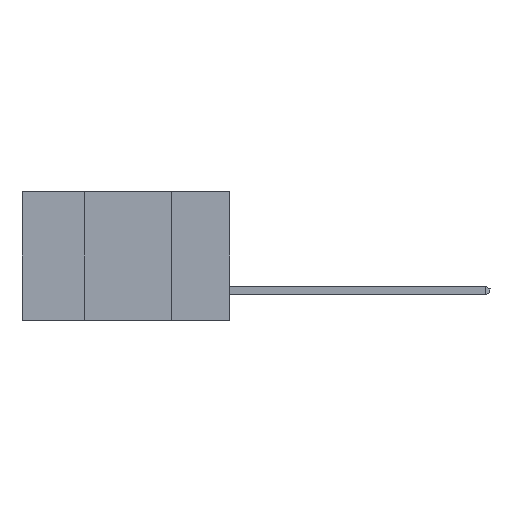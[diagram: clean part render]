
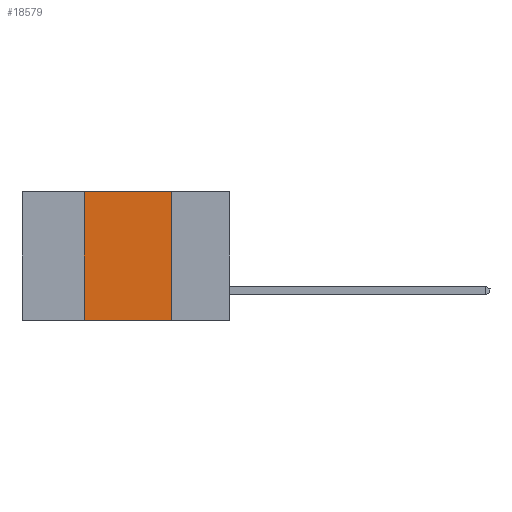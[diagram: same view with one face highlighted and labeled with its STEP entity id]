
A CAD part, left-side view. The second image highlights one B-rep face of the part: STEP entity #18579.
In plain terms, the highlighted planar face has unit normal (-1, 0, 0).
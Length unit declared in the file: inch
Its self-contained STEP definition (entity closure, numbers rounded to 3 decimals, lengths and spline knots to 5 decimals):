
#257 = FACE_OUTER_BOUND ( 'NONE', #25144, .T. ) ;
#737 = CARTESIAN_POINT ( 'NONE',  ( 0., 0.6, -0.37 ) ) ;
#833 = LINE ( 'NONE', #20467, #21780 ) ;
#2364 = DIRECTION ( 'NONE',  ( 0., 0., -1. ) ) ;
#2722 = LINE ( 'NONE', #20997, #23050 ) ;
#3212 = CARTESIAN_POINT ( 'NONE',  ( 0., 0.6, 0. ) ) ;
#3334 = DIRECTION ( 'NONE',  ( 0., -1., 0. ) ) ;
#3952 = VERTEX_POINT ( 'NONE', #21026 ) ;
#5825 = CARTESIAN_POINT ( 'NONE',  ( 0., 0.17, 0. ) ) ;
#6505 = CARTESIAN_POINT ( 'NONE',  ( 0., 0.42, -0.37 ) ) ;
#6586 = DIRECTION ( 'NONE',  ( 0., -1., 0. ) ) ;
#8256 = CARTESIAN_POINT ( 'NONE',  ( 0., 0.6, 0. ) ) ;
#10914 = VERTEX_POINT ( 'NONE', #5825 ) ;
#11206 = VERTEX_POINT ( 'NONE', #25024 ) ;
#11713 = AXIS2_PLACEMENT_3D ( 'NONE', #8256, #20779, #2364 ) ;
#12486 = VERTEX_POINT ( 'NONE', #6505 ) ;
#12836 = DIRECTION ( 'NONE',  ( 0., 0., -1. ) ) ;
#14929 = ORIENTED_EDGE ( 'NONE', *, *, #26139, .F. ) ;
#15029 = ORIENTED_EDGE ( 'NONE', *, *, #22091, .T. ) ;
#15104 = DIRECTION ( 'NONE',  ( 0., 0., 1. ) ) ;
#17114 = VECTOR ( 'NONE', #3334, 39.37008 ) ;
#18579 = ADVANCED_FACE ( 'NONE', ( #257 ), #22770, .F. ) ;
#18668 = LINE ( 'NONE', #3212, #17114 ) ;
#19961 = ORIENTED_EDGE ( 'NONE', *, *, #24309, .F. ) ;
#19999 = ORIENTED_EDGE ( 'NONE', *, *, #23776, .F. ) ;
#20467 = CARTESIAN_POINT ( 'NONE',  ( 0., 0.42, -0.37 ) ) ;
#20779 = DIRECTION ( 'NONE',  ( 1., 0., 0. ) ) ;
#20997 = CARTESIAN_POINT ( 'NONE',  ( 0., 0.17, -0.37 ) ) ;
#21001 = LINE ( 'NONE', #737, #22053 ) ;
#21026 = CARTESIAN_POINT ( 'NONE',  ( 0., 0.17, -0.37 ) ) ;
#21780 = VECTOR ( 'NONE', #15104, 39.37008 ) ;
#22053 = VECTOR ( 'NONE', #6586, 39.37008 ) ;
#22091 = EDGE_CURVE ( 'NONE', #12486, #3952, #21001, .T. ) ;
#22770 = PLANE ( 'NONE',  #11713 ) ;
#23050 = VECTOR ( 'NONE', #12836, 39.37008 ) ;
#23776 = EDGE_CURVE ( 'NONE', #12486, #11206, #833, .T. ) ;
#24309 = EDGE_CURVE ( 'NONE', #11206, #10914, #18668, .T. ) ;
#25024 = CARTESIAN_POINT ( 'NONE',  ( 0., 0.42, 0. ) ) ;
#25144 = EDGE_LOOP ( 'NONE', ( #14929, #19961, #19999, #15029 ) ) ;
#26139 = EDGE_CURVE ( 'NONE', #10914, #3952, #2722, .T. ) ;
